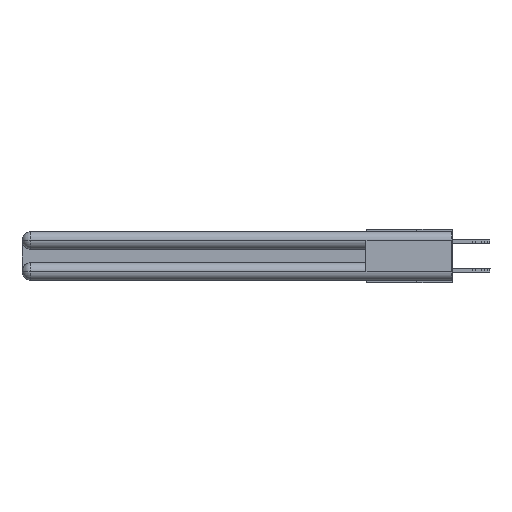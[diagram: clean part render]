
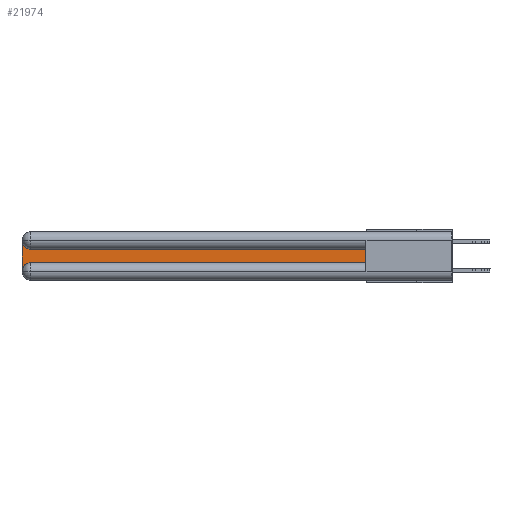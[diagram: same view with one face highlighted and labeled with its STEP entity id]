
A CAD part, left-side view. The second image highlights one B-rep face of the part: STEP entity #21974.
In plain terms, the highlighted planar face has unit normal (-1, 0, 0).
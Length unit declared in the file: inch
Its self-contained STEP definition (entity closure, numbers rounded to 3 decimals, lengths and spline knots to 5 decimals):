
#49 = DIRECTION ( 'NONE',  ( 0., 0., -1. ) ) ;
#213 = CARTESIAN_POINT ( 'NONE',  ( 0.075, 0.6, -0.1225 ) ) ;
#261 = CARTESIAN_POINT ( 'NONE',  ( 0.075, 0.6, -0.2175 ) ) ;
#1135 = LINE ( 'NONE', #15108, #25357 ) ;
#1924 = EDGE_CURVE ( 'NONE', #21331, #13569, #5934, .T. ) ;
#2348 = ORIENTED_EDGE ( 'NONE', *, *, #4743, .T. ) ;
#3025 = DIRECTION ( 'NONE',  ( 0., 0., -1. ) ) ;
#3188 = DIRECTION ( 'NONE',  ( 1., 0., 0. ) ) ;
#3771 = EDGE_CURVE ( 'NONE', #18345, #15329, #1135, .T. ) ;
#4132 = CARTESIAN_POINT ( 'NONE',  ( 0.075, 2.94, -0.0625 ) ) ;
#4340 = EDGE_CURVE ( 'NONE', #26757, #18345, #21982, .T. ) ;
#4743 = EDGE_CURVE ( 'NONE', #13569, #26757, #17607, .T. ) ;
#5007 = LINE ( 'NONE', #28361, #28933 ) ;
#5519 = DIRECTION ( 'NONE',  ( 0., 0., -1. ) ) ;
#5934 = LINE ( 'NONE', #22197, #29865 ) ;
#6537 = AXIS2_PLACEMENT_3D ( 'NONE', #21656, #3188, #7920 ) ;
#6943 = ORIENTED_EDGE ( 'NONE', *, *, #28927, .T. ) ;
#7159 = CARTESIAN_POINT ( 'NONE',  ( 0.075, 0.6, -0.1225 ) ) ;
#7920 = DIRECTION ( 'NONE',  ( 0., 0., -1. ) ) ;
#10180 = EDGE_CURVE ( 'NONE', #15329, #21172, #23034, .T. ) ;
#10385 = EDGE_LOOP ( 'NONE', ( #2348, #26490, #17325, #15262, #6943, #27126 ) ) ;
#10997 = CARTESIAN_POINT ( 'NONE',  ( 0.075, 2.94, -0.2175 ) ) ;
#13070 = DIRECTION ( 'NONE',  ( 0., 0., 1. ) ) ;
#13569 = VERTEX_POINT ( 'NONE', #7159 ) ;
#15108 = CARTESIAN_POINT ( 'NONE',  ( 0.075, 3., -0.2175 ) ) ;
#15262 = ORIENTED_EDGE ( 'NONE', *, *, #10180, .T. ) ;
#15329 = VERTEX_POINT ( 'NONE', #24312 ) ;
#16803 = CARTESIAN_POINT ( 'NONE',  ( 0.075, 2.94, -0.2775 ) ) ;
#17325 = ORIENTED_EDGE ( 'NONE', *, *, #3771, .T. ) ;
#17607 = LINE ( 'NONE', #213, #23074 ) ;
#17700 = AXIS2_PLACEMENT_3D ( 'NONE', #16803, #23827, #3025 ) ;
#18003 = CARTESIAN_POINT ( 'NONE',  ( 0.075, 2.94, -0.1225 ) ) ;
#18046 = DIRECTION ( 'NONE',  ( 1., 0., 0. ) ) ;
#18345 = VERTEX_POINT ( 'NONE', #18395 ) ;
#18395 = CARTESIAN_POINT ( 'NONE',  ( 0.075, 3., -0.0625 ) ) ;
#21172 = VERTEX_POINT ( 'NONE', #10997 ) ;
#21331 = VERTEX_POINT ( 'NONE', #261 ) ;
#21656 = CARTESIAN_POINT ( 'NONE',  ( 0.075, 3., -0.1225 ) ) ;
#21974 = ADVANCED_FACE ( 'NONE', ( #25843 ), #23988, .F. ) ;
#21982 = CIRCLE ( 'NONE', #26552, 0.06 ) ;
#22197 = CARTESIAN_POINT ( 'NONE',  ( 0.075, 0.6, -0.2175 ) ) ;
#23034 = CIRCLE ( 'NONE', #17700, 0.06 ) ;
#23074 = VECTOR ( 'NONE', #25501, 39.37008 ) ;
#23827 = DIRECTION ( 'NONE',  ( 1., 0., 0. ) ) ;
#23988 = PLANE ( 'NONE',  #6537 ) ;
#24312 = CARTESIAN_POINT ( 'NONE',  ( 0.075, 3., -0.2775 ) ) ;
#25357 = VECTOR ( 'NONE', #5519, 39.37008 ) ;
#25501 = DIRECTION ( 'NONE',  ( 0., 1., 0. ) ) ;
#25613 = DIRECTION ( 'NONE',  ( 0., -1., 0. ) ) ;
#25843 = FACE_OUTER_BOUND ( 'NONE', #10385, .T. ) ;
#26490 = ORIENTED_EDGE ( 'NONE', *, *, #4340, .T. ) ;
#26552 = AXIS2_PLACEMENT_3D ( 'NONE', #4132, #18046, #49 ) ;
#26757 = VERTEX_POINT ( 'NONE', #18003 ) ;
#27126 = ORIENTED_EDGE ( 'NONE', *, *, #1924, .T. ) ;
#28361 = CARTESIAN_POINT ( 'NONE',  ( 0.075, 0.6, -0.2175 ) ) ;
#28927 = EDGE_CURVE ( 'NONE', #21172, #21331, #5007, .T. ) ;
#28933 = VECTOR ( 'NONE', #25613, 39.37008 ) ;
#29865 = VECTOR ( 'NONE', #13070, 39.37008 ) ;
